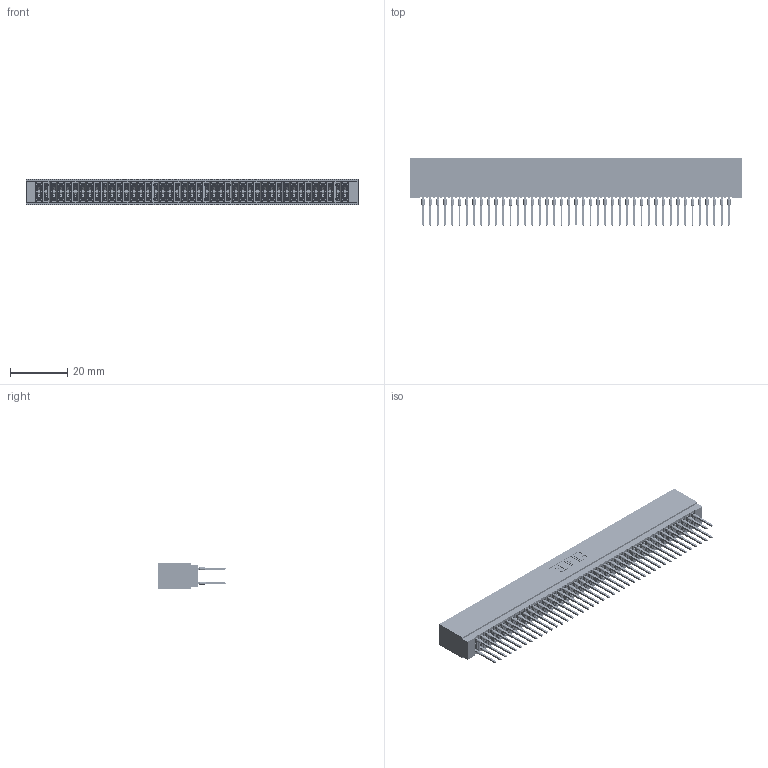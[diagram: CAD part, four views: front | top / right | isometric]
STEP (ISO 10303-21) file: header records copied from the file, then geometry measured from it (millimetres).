
FILE_DESCRIPTION (( 'STEP AP203' ), '1' );
FILE_NAME ('725-086-522-201.STEP', '2026-02-24T19:16:20', ( '' ), ( '' ), 'SwSTEP 2.0', 'SolidWorks 2023', '' );
FILE_SCHEMA (( 'CONFIG_CONTROL_DESIGN' ));
Length unit declared in the file: millimetre
Products named in the file (3): 725 Part_Insulator Option - 01; 745-292-001_522; 725-086-522-201
Assembly tree (87 placements, depth 2):
  725-086-522-201
    725 Part_Insulator Option - 01
    745-292-001_522  x86
Bounding box: 115.82 x 23.51 x 8.89 mm (x, y, z)
Volume: 9271 mm3; surface area: 19920 mm2
Topology: 87 solids, 87 shells, 7792 faces, 20937 edges, 13154 vertices
Faces by surface type: plane 4011, bspline 1720, cylinder 1545, torus 516
Entity records: 72219 total; most frequent: CARTESIAN_POINT 13027, ORIENTED_EDGE 12464, DIRECTION 10890, EDGE_CURVE 6232, LINE 5792, VECTOR 5792, VERTEX_POINT 3974, AXIS2_PLACEMENT_3D 2549
